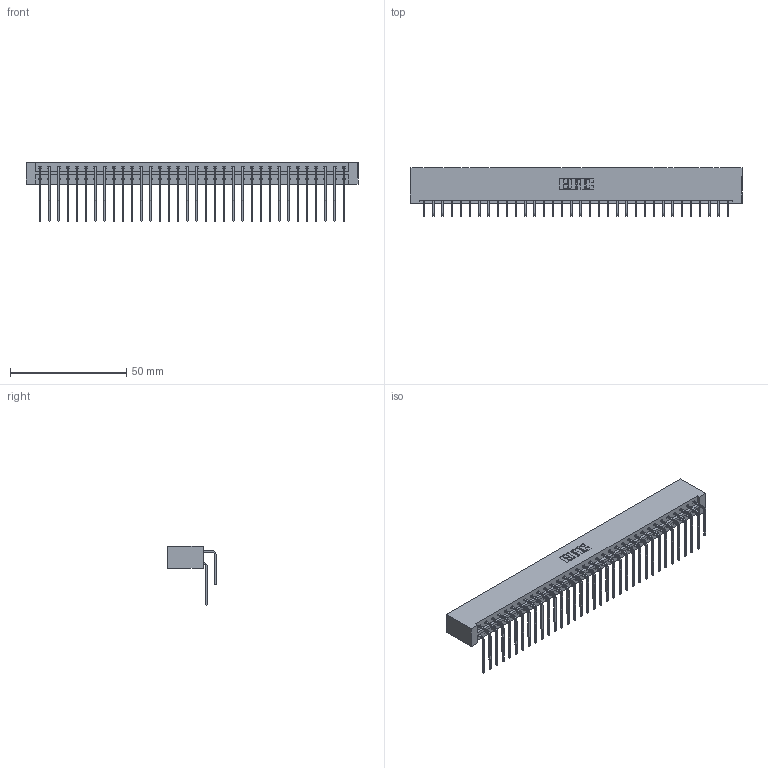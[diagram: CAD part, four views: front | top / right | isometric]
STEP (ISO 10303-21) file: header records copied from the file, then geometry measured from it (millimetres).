
FILE_DESCRIPTION (( 'STEP AP203' ), '1' );
FILE_NAME ('833-068-559-201.STEP', '2020-06-05T11:25:30', ( '' ), ( '' ), 'SwSTEP 2.0', 'SolidWorks 2020', '' );
FILE_SCHEMA (( 'CONFIG_CONTROL_DESIGN' ));
Length unit declared in the file: inch
Products named in the file (4): 345-292-001_558 559 Tail - 1; 345-292-001_559 Tail - 2; 833 Part_Lugless; 833-068-559-201
Assembly tree (69 placements, depth 2):
  833-068-559-201
    833 Part_Lugless
    345-292-001_558 559 Tail - 1  x34
    345-292-001_559 Tail - 2  x34
Bounding box: 142.98 x 20.9 x 25.53 mm (x, y, z)
Volume: 15546.8 mm3; surface area: 20272.5 mm2
Topology: 69 solids, 69 shells, 3778 faces, 11235 edges, 7398 vertices
Faces by surface type: plane 2650, cylinder 1128
Entity records: 24415 total; most frequent: CARTESIAN_POINT 4105, ORIENTED_EDGE 3990, DIRECTION 3495, EDGE_CURVE 1995, VECTOR 1835, LINE 1835, VERTEX_POINT 1326, AXIS2_PLACEMENT_3D 830
